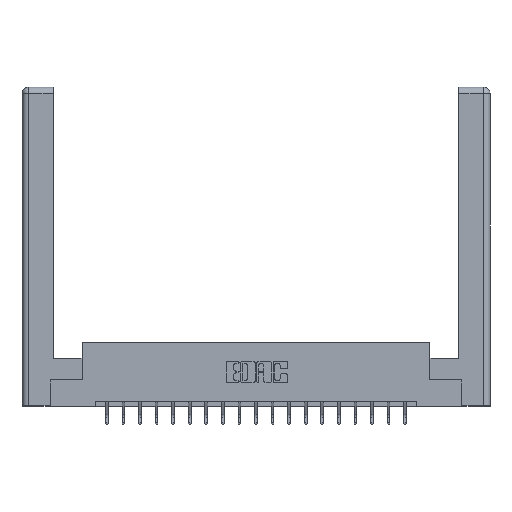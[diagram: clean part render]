
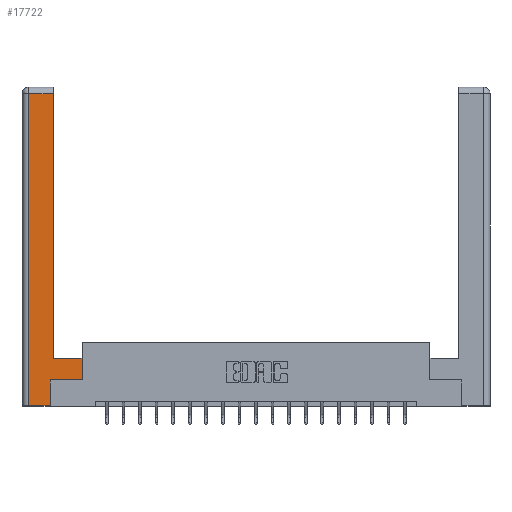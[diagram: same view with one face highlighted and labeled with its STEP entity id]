
A CAD part, top view. The second image highlights one B-rep face of the part: STEP entity #17722.
In plain terms, the highlighted planar face has unit normal (0, 0, 1).
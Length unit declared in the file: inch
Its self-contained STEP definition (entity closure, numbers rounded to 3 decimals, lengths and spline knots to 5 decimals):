
#451 = DIRECTION ( 'NONE',  ( 0., 1., 0. ) ) ;
#633 = LINE ( 'NONE', #16805, #9629 ) ;
#788 = VERTEX_POINT ( 'NONE', #16037 ) ;
#1280 = VERTEX_POINT ( 'NONE', #7959 ) ;
#1669 = EDGE_CURVE ( 'NONE', #16937, #788, #633, .T. ) ;
#2031 = VECTOR ( 'NONE', #16617, 39.37008 ) ;
#2273 = DIRECTION ( 'NONE',  ( -1., 0., 0. ) ) ;
#2903 = CARTESIAN_POINT ( 'NONE',  ( 0.265, 0., 0. ) ) ;
#3125 = ORIENTED_EDGE ( 'NONE', *, *, #3459, .T. ) ;
#3127 = ORIENTED_EDGE ( 'NONE', *, *, #11535, .T. ) ;
#3459 = EDGE_CURVE ( 'NONE', #8403, #17962, #18010, .T. ) ;
#3621 = ORIENTED_EDGE ( 'NONE', *, *, #13297, .T. ) ;
#3891 = DIRECTION ( 'NONE',  ( 0., 1., 0. ) ) ;
#4459 = LINE ( 'NONE', #10367, #11437 ) ;
#4764 = DIRECTION ( 'NONE',  ( 0., -1., 0. ) ) ;
#5589 = ORIENTED_EDGE ( 'NONE', *, *, #19076, .T. ) ;
#6417 = CARTESIAN_POINT ( 'NONE',  ( 0.565, 0.245, 0. ) ) ;
#6719 = VECTOR ( 'NONE', #16972, 39.37008 ) ;
#7086 = VERTEX_POINT ( 'NONE', #9619 ) ;
#7087 = CARTESIAN_POINT ( 'NONE',  ( 0.0615, 2.94, 0. ) ) ;
#7223 = LINE ( 'NONE', #12188, #6719 ) ;
#7235 = CARTESIAN_POINT ( 'NONE',  ( 0., 0., 0. ) ) ;
#7811 = LINE ( 'NONE', #11547, #12040 ) ;
#7959 = CARTESIAN_POINT ( 'NONE',  ( 0.265, 0.245, 0. ) ) ;
#8403 = VERTEX_POINT ( 'NONE', #10004 ) ;
#8653 = CARTESIAN_POINT ( 'NONE',  ( 0.565, 0.45, 0. ) ) ;
#8748 = VECTOR ( 'NONE', #19710, 39.37008 ) ;
#9619 = CARTESIAN_POINT ( 'NONE',  ( 0.295, 2.94, 0. ) ) ;
#9629 = VECTOR ( 'NONE', #2273, 39.37008 ) ;
#10004 = CARTESIAN_POINT ( 'NONE',  ( 0.0615, 0., 0. ) ) ;
#10276 = CARTESIAN_POINT ( 'NONE',  ( 0.565, 0.45, 0. ) ) ;
#10367 = CARTESIAN_POINT ( 'NONE',  ( 0.295, 3., 0. ) ) ;
#10483 = CARTESIAN_POINT ( 'NONE',  ( 0.265, 0., 0. ) ) ;
#10503 = LINE ( 'NONE', #16681, #2031 ) ;
#10619 = EDGE_CURVE ( 'NONE', #7086, #12933, #10503, .T. ) ;
#10627 = ORIENTED_EDGE ( 'NONE', *, *, #1669, .T. ) ;
#10976 = ORIENTED_EDGE ( 'NONE', *, *, #19675, .T. ) ;
#11264 = ORIENTED_EDGE ( 'NONE', *, *, #10619, .T. ) ;
#11437 = VECTOR ( 'NONE', #3891, 39.37008 ) ;
#11535 = EDGE_CURVE ( 'NONE', #17962, #1280, #7811, .T. ) ;
#11547 = CARTESIAN_POINT ( 'NONE',  ( 0.265, 0.245, 0. ) ) ;
#12035 = ORIENTED_EDGE ( 'NONE', *, *, #18920, .T. ) ;
#12040 = VECTOR ( 'NONE', #451, 39.37008 ) ;
#12188 = CARTESIAN_POINT ( 'NONE',  ( 0.565, 0.245, 0. ) ) ;
#12707 = LINE ( 'NONE', #8653, #8748 ) ;
#12763 = CARTESIAN_POINT ( 'NONE',  ( 0.0615, 0., 0. ) ) ;
#12933 = VERTEX_POINT ( 'NONE', #7087 ) ;
#13297 = EDGE_CURVE ( 'NONE', #1280, #14844, #7223, .T. ) ;
#13452 = VECTOR ( 'NONE', #4764, 39.37008 ) ;
#13643 = PLANE ( 'NONE',  #16449 ) ;
#14314 = DIRECTION ( 'NONE',  ( 1., 0., 0. ) ) ;
#14844 = VERTEX_POINT ( 'NONE', #6417 ) ;
#15259 = VECTOR ( 'NONE', #14314, 39.37008 ) ;
#15728 = FACE_OUTER_BOUND ( 'NONE', #17572, .T. ) ;
#16037 = CARTESIAN_POINT ( 'NONE',  ( 0.295, 0.45, 0. ) ) ;
#16449 = AXIS2_PLACEMENT_3D ( 'NONE', #7235, #19930, #18479 ) ;
#16617 = DIRECTION ( 'NONE',  ( -1., 0., 0. ) ) ;
#16681 = CARTESIAN_POINT ( 'NONE',  ( 0.0615, 2.94, 0. ) ) ;
#16805 = CARTESIAN_POINT ( 'NONE',  ( 0.295, 0.45, 0. ) ) ;
#16937 = VERTEX_POINT ( 'NONE', #10276 ) ;
#16972 = DIRECTION ( 'NONE',  ( 1., 0., 0. ) ) ;
#17572 = EDGE_LOOP ( 'NONE', ( #10976, #11264, #5589, #3125, #3127, #3621, #12035, #10627 ) ) ;
#17722 = ADVANCED_FACE ( 'NONE', ( #15728 ), #13643, .F. ) ;
#17962 = VERTEX_POINT ( 'NONE', #2903 ) ;
#18010 = LINE ( 'NONE', #10483, #15259 ) ;
#18406 = LINE ( 'NONE', #12763, #13452 ) ;
#18479 = DIRECTION ( 'NONE',  ( -1., 0., 0. ) ) ;
#18920 = EDGE_CURVE ( 'NONE', #14844, #16937, #12707, .T. ) ;
#19076 = EDGE_CURVE ( 'NONE', #12933, #8403, #18406, .T. ) ;
#19675 = EDGE_CURVE ( 'NONE', #788, #7086, #4459, .T. ) ;
#19710 = DIRECTION ( 'NONE',  ( 0., 1., 0. ) ) ;
#19930 = DIRECTION ( 'NONE',  ( 0., 0., -1. ) ) ;
